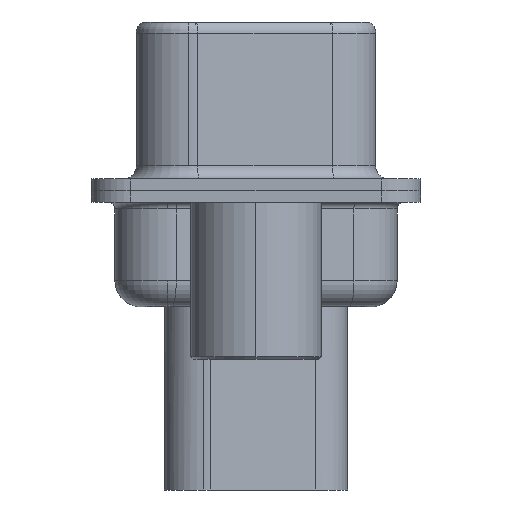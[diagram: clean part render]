
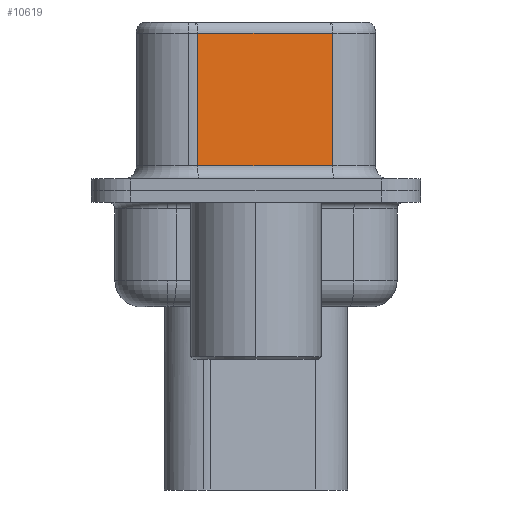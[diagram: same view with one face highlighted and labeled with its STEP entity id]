
A CAD part, left-side view. The second image highlights one B-rep face of the part: STEP entity #10619.
In plain terms, the highlighted planar face has unit normal (-0.985, -0.174, 0).
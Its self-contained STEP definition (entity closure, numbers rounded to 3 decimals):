
#269 = FACE_OUTER_BOUND ( 'NONE', #22349, .T. ) ;
#411 = CARTESIAN_POINT ( 'NONE',  ( 4.58, -2.927, 6.52 ) ) ;
#1358 = CARTESIAN_POINT ( 'NONE',  ( 3.67, 2.233, 0.95 ) ) ;
#2259 = EDGE_CURVE ( 'NONE', #11530, #17986, #10472, .T. ) ;
#2761 = DIRECTION ( 'NONE',  ( -0.174, 0.985, 0. ) ) ;
#3645 = CARTESIAN_POINT ( 'NONE',  ( 4.58, -2.927, 6.52 ) ) ;
#3811 = VECTOR ( 'NONE', #21613, 1000. ) ;
#4524 = EDGE_CURVE ( 'NONE', #19720, #16153, #15408, .T. ) ;
#5395 = CARTESIAN_POINT ( 'NONE',  ( 4.58, -2.927, 6.02 ) ) ;
#5766 = CARTESIAN_POINT ( 'NONE',  ( 3.67, 2.233, 6.02 ) ) ;
#6886 = EDGE_CURVE ( 'NONE', #16153, #11530, #7339, .T. ) ;
#7339 = LINE ( 'NONE', #12824, #3811 ) ;
#7436 = DIRECTION ( 'NONE',  ( 0., 0., -1. ) ) ;
#8033 = CARTESIAN_POINT ( 'NONE',  ( 4.58, -2.927, 6.02 ) ) ;
#9156 = ORIENTED_EDGE ( 'NONE', *, *, #6886, .T. ) ;
#10043 = AXIS2_PLACEMENT_3D ( 'NONE', #3645, #21263, #10693 ) ;
#10169 = VECTOR ( 'NONE', #2761, 1000. ) ;
#10472 = LINE ( 'NONE', #19188, #14607 ) ;
#10619 = ADVANCED_FACE ( 'NONE', ( #269 ), #10621, .F. ) ;
#10621 = PLANE ( 'NONE',  #10043 ) ;
#10693 = DIRECTION ( 'NONE',  ( -0.174, 0.985, 0. ) ) ;
#10698 = LINE ( 'NONE', #411, #20088 ) ;
#11530 = VERTEX_POINT ( 'NONE', #1358 ) ;
#12824 = CARTESIAN_POINT ( 'NONE',  ( 3.67, 2.233, 6.52 ) ) ;
#13367 = ORIENTED_EDGE ( 'NONE', *, *, #4524, .T. ) ;
#14607 = VECTOR ( 'NONE', #20057, 1000. ) ;
#15140 = CARTESIAN_POINT ( 'NONE',  ( 4.58, -2.927, 0.95 ) ) ;
#15408 = LINE ( 'NONE', #5395, #10169 ) ;
#16127 = EDGE_CURVE ( 'NONE', #19720, #17986, #10698, .T. ) ;
#16153 = VERTEX_POINT ( 'NONE', #5766 ) ;
#17132 = ORIENTED_EDGE ( 'NONE', *, *, #2259, .T. ) ;
#17986 = VERTEX_POINT ( 'NONE', #15140 ) ;
#18285 = ORIENTED_EDGE ( 'NONE', *, *, #16127, .F. ) ;
#19188 = CARTESIAN_POINT ( 'NONE',  ( 4.58, -2.927, 0.95 ) ) ;
#19720 = VERTEX_POINT ( 'NONE', #8033 ) ;
#20057 = DIRECTION ( 'NONE',  ( 0.174, -0.985, 0. ) ) ;
#20088 = VECTOR ( 'NONE', #7436, 1000. ) ;
#21263 = DIRECTION ( 'NONE',  ( 0.985, 0.174, 0. ) ) ;
#21613 = DIRECTION ( 'NONE',  ( 0., 0., -1. ) ) ;
#22349 = EDGE_LOOP ( 'NONE', ( #18285, #13367, #9156, #17132 ) ) ;
